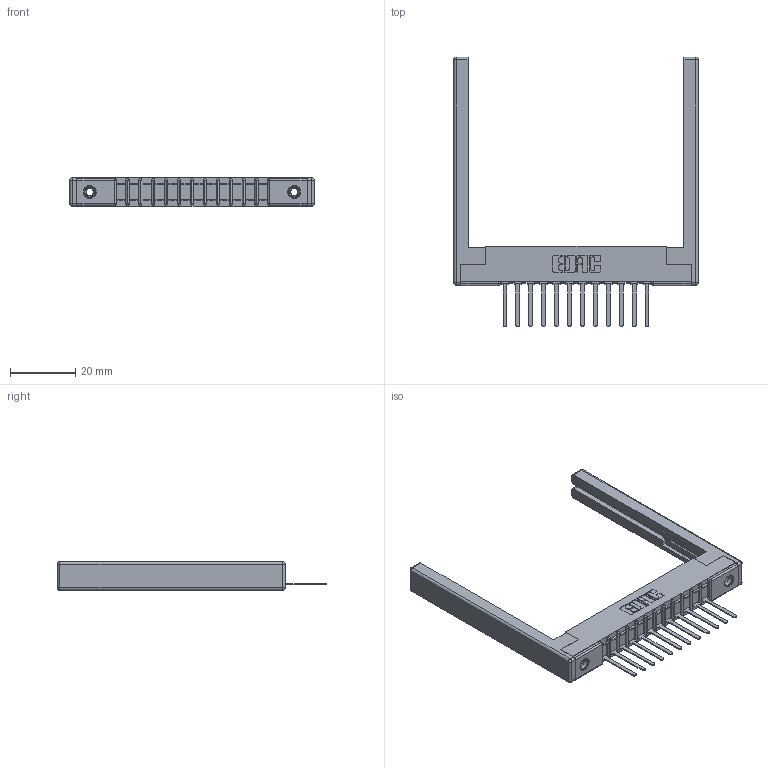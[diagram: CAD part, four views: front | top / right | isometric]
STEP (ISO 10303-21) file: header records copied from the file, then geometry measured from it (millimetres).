
FILE_DESCRIPTION (( 'STEP AP203' ), '1' );
FILE_NAME ('357-012-541-168.STEP', '2019-09-16T19:14:02', ( '' ), ( '' ), 'SwSTEP 2.0', 'SolidWorks 2016', '' );
FILE_SCHEMA (( 'CONFIG_CONTROL_DESIGN' ));
Length unit declared in the file: inch
Products named in the file (5): 345-250-001_345-250-001-102; 307-290-002_541; 307 Part_.156 Dia Mounting Holes; 307-220-068; 357-012-541-168
Assembly tree (17 placements, depth 2):
  357-012-541-168
    307 Part_.156 Dia Mounting Holes
    307-290-002_541  x12
    307-220-068  x2
    345-250-001_345-250-001-102  x2
Bounding box: 74.98 x 82.55 x 8.71 mm (x, y, z)
Volume: 9537.5 mm3; surface area: 12724.5 mm2
Topology: 17 solids, 17 shells, 1173 faces, 3497 edges, 2274 vertices
Faces by surface type: plane 698, cylinder 425, sphere 34, cone 12, torus 4
Entity records: 17463 total; most frequent: CARTESIAN_POINT 2905, ORIENTED_EDGE 2884, DIRECTION 2854, EDGE_CURVE 1442, VECTOR 1088, LINE 1088, VERTEX_POINT 934, AXIS2_PLACEMENT_3D 883
